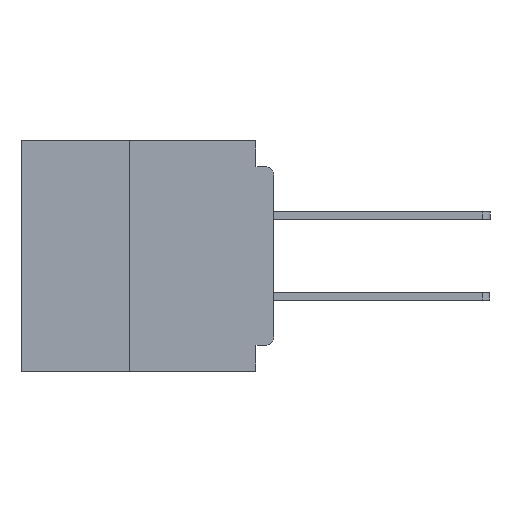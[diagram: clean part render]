
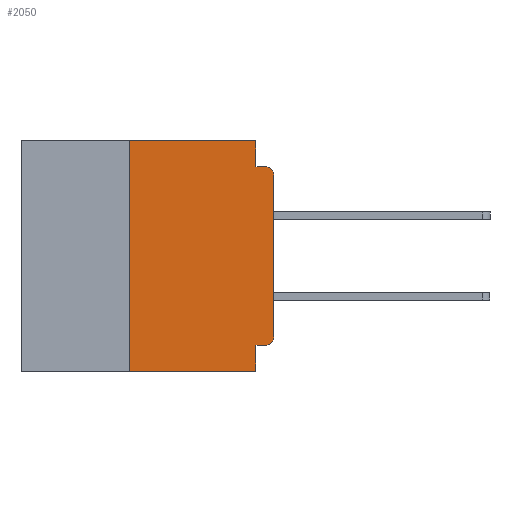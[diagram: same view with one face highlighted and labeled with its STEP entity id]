
A CAD part, left-side view. The second image highlights one B-rep face of the part: STEP entity #2050.
In plain terms, the highlighted planar face has unit normal (-1, 0, 0).
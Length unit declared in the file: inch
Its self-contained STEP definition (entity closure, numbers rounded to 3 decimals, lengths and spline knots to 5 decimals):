
#98 = ORIENTED_EDGE ( 'NONE', *, *, #4090, .F. ) ;
#127 = DIRECTION ( 'NONE',  ( 0., 0., -1. ) ) ;
#217 = ORIENTED_EDGE ( 'NONE', *, *, #2578, .F. ) ;
#550 = VECTOR ( 'NONE', #31088, 39.37008 ) ;
#846 = AXIS2_PLACEMENT_3D ( 'NONE', #28073, #9573, #31152 ) ;
#1230 = CARTESIAN_POINT ( 'NONE',  ( 0., 0.25, -0.4 ) ) ;
#1253 = DIRECTION ( 'NONE',  ( -1., 0., 0. ) ) ;
#1384 = CARTESIAN_POINT ( 'NONE',  ( 0., 0.031, 0. ) ) ;
#2050 = ADVANCED_FACE ( 'NONE', ( #7716 ), #38795, .F. ) ;
#2215 = LINE ( 'NONE', #36433, #9604 ) ;
#2407 = LINE ( 'NONE', #20081, #9781 ) ;
#2578 = EDGE_CURVE ( 'NONE', #10617, #13691, #7676, .T. ) ;
#3051 = ORIENTED_EDGE ( 'NONE', *, *, #37439, .F. ) ;
#3225 = LINE ( 'NONE', #30528, #18811 ) ;
#3378 = EDGE_CURVE ( 'NONE', #12482, #22680, #3225, .T. ) ;
#3614 = DIRECTION ( 'NONE',  ( 0., -1., 0. ) ) ;
#3748 = CARTESIAN_POINT ( 'NONE',  ( 0., 0.437, -0.4 ) ) ;
#4090 = EDGE_CURVE ( 'NONE', #13691, #37470, #2215, .T. ) ;
#4190 = ORIENTED_EDGE ( 'NONE', *, *, #32183, .F. ) ;
#5333 = AXIS2_PLACEMENT_3D ( 'NONE', #38544, #37635, #37465 ) ;
#5534 = CARTESIAN_POINT ( 'NONE',  ( 0., 0.031, -0.045 ) ) ;
#5649 = EDGE_CURVE ( 'NONE', #20235, #22680, #22385, .T. ) ;
#6206 = CARTESIAN_POINT ( 'NONE',  ( 0., 0., -0.34 ) ) ;
#7106 = VERTEX_POINT ( 'NONE', #23321 ) ;
#7661 = CARTESIAN_POINT ( 'NONE',  ( 0., 0.031, -0.355 ) ) ;
#7676 = LINE ( 'NONE', #1384, #39432 ) ;
#7716 = FACE_OUTER_BOUND ( 'NONE', #10513, .T. ) ;
#7904 = VECTOR ( 'NONE', #8772, 39.37008 ) ;
#8772 = DIRECTION ( 'NONE',  ( 0., 1., 0. ) ) ;
#8949 = EDGE_CURVE ( 'NONE', #23092, #37384, #13415, .T. ) ;
#9573 = DIRECTION ( 'NONE',  ( -1., 0., 0. ) ) ;
#9604 = VECTOR ( 'NONE', #36478, 39.37008 ) ;
#9781 = VECTOR ( 'NONE', #23219, 39.37008 ) ;
#10513 = EDGE_LOOP ( 'NONE', ( #31265, #31944, #98, #217, #3051, #4190, #15500, #16749, #26883, #30618 ) ) ;
#10617 = VERTEX_POINT ( 'NONE', #28189 ) ;
#12482 = VERTEX_POINT ( 'NONE', #7661 ) ;
#12803 = CARTESIAN_POINT ( 'NONE',  ( 0., 0.437, 0. ) ) ;
#13415 = CIRCLE ( 'NONE', #17478, 0.015 ) ;
#13691 = VERTEX_POINT ( 'NONE', #5534 ) ;
#15500 = ORIENTED_EDGE ( 'NONE', *, *, #5649, .T. ) ;
#15955 = CARTESIAN_POINT ( 'NONE',  ( 0., 0., 0. ) ) ;
#16749 = ORIENTED_EDGE ( 'NONE', *, *, #3378, .F. ) ;
#17199 = LINE ( 'NONE', #12803, #550 ) ;
#17478 = AXIS2_PLACEMENT_3D ( 'NONE', #19920, #1253, #23064 ) ;
#18811 = VECTOR ( 'NONE', #30619, 39.37008 ) ;
#19920 = CARTESIAN_POINT ( 'NONE',  ( 0., 0.015, -0.34 ) ) ;
#20081 = CARTESIAN_POINT ( 'NONE',  ( 0., 0.25, -0.4 ) ) ;
#20235 = VERTEX_POINT ( 'NONE', #1230 ) ;
#21262 = EDGE_CURVE ( 'NONE', #37384, #7106, #33450, .T. ) ;
#22385 = LINE ( 'NONE', #3748, #37652 ) ;
#22680 = VERTEX_POINT ( 'NONE', #34277 ) ;
#23064 = DIRECTION ( 'NONE',  ( 0., 0., -1. ) ) ;
#23092 = VERTEX_POINT ( 'NONE', #36787 ) ;
#23219 = DIRECTION ( 'NONE',  ( 0., 0., 1. ) ) ;
#23321 = CARTESIAN_POINT ( 'NONE',  ( 0., 0., -0.06 ) ) ;
#25291 = DIRECTION ( 'NONE',  ( 0., 0., 1. ) ) ;
#25359 = CARTESIAN_POINT ( 'NONE',  ( 0., 0.015, -0.045 ) ) ;
#25415 = LINE ( 'NONE', #33268, #7904 ) ;
#26330 = VECTOR ( 'NONE', #25291, 39.37008 ) ;
#26569 = VERTEX_POINT ( 'NONE', #32870 ) ;
#26883 = ORIENTED_EDGE ( 'NONE', *, *, #37883, .F. ) ;
#27684 = CIRCLE ( 'NONE', #846, 0.015 ) ;
#28073 = CARTESIAN_POINT ( 'NONE',  ( 0., 0.015, -0.06 ) ) ;
#28189 = CARTESIAN_POINT ( 'NONE',  ( 0., 0.031, 0. ) ) ;
#30528 = CARTESIAN_POINT ( 'NONE',  ( 0., 0.031, -0.4 ) ) ;
#30618 = ORIENTED_EDGE ( 'NONE', *, *, #8949, .T. ) ;
#30619 = DIRECTION ( 'NONE',  ( 0., 0., -1. ) ) ;
#31088 = DIRECTION ( 'NONE',  ( 0., -1., 0. ) ) ;
#31152 = DIRECTION ( 'NONE',  ( 0., 0., -1. ) ) ;
#31265 = ORIENTED_EDGE ( 'NONE', *, *, #21262, .T. ) ;
#31901 = EDGE_CURVE ( 'NONE', #7106, #37470, #27684, .T. ) ;
#31944 = ORIENTED_EDGE ( 'NONE', *, *, #31901, .T. ) ;
#32183 = EDGE_CURVE ( 'NONE', #20235, #26569, #2407, .T. ) ;
#32870 = CARTESIAN_POINT ( 'NONE',  ( 0., 0.25, 0. ) ) ;
#33268 = CARTESIAN_POINT ( 'NONE',  ( 0., 0., -0.355 ) ) ;
#33450 = LINE ( 'NONE', #15955, #26330 ) ;
#34277 = CARTESIAN_POINT ( 'NONE',  ( 0., 0.031, -0.4 ) ) ;
#36433 = CARTESIAN_POINT ( 'NONE',  ( 0., 0., -0.045 ) ) ;
#36478 = DIRECTION ( 'NONE',  ( 0., -1., 0. ) ) ;
#36787 = CARTESIAN_POINT ( 'NONE',  ( 0., 0.015, -0.355 ) ) ;
#37384 = VERTEX_POINT ( 'NONE', #6206 ) ;
#37439 = EDGE_CURVE ( 'NONE', #26569, #10617, #17199, .T. ) ;
#37465 = DIRECTION ( 'NONE',  ( 0., 0., -1. ) ) ;
#37470 = VERTEX_POINT ( 'NONE', #25359 ) ;
#37635 = DIRECTION ( 'NONE',  ( 1., 0., 0. ) ) ;
#37652 = VECTOR ( 'NONE', #3614, 39.37008 ) ;
#37883 = EDGE_CURVE ( 'NONE', #23092, #12482, #25415, .T. ) ;
#38544 = CARTESIAN_POINT ( 'NONE',  ( 0., 0.437, 0. ) ) ;
#38795 = PLANE ( 'NONE',  #5333 ) ;
#39432 = VECTOR ( 'NONE', #127, 39.37008 ) ;
